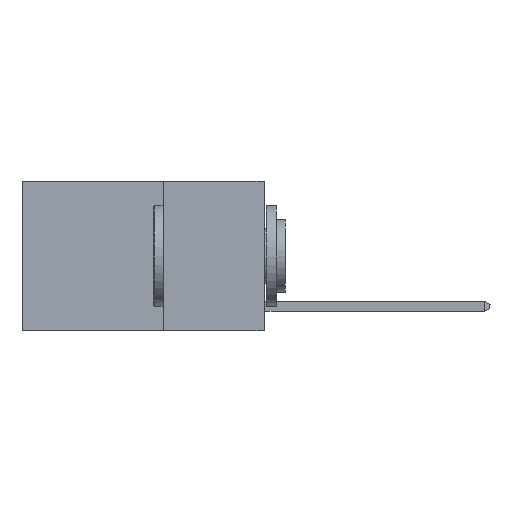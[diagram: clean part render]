
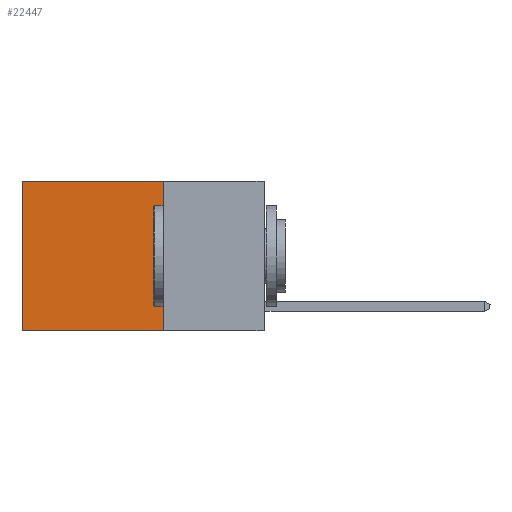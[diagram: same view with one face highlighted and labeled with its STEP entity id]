
A CAD part, left-side view. The second image highlights one B-rep face of the part: STEP entity #22447.
In plain terms, the highlighted planar face has unit normal (-1, 0, 0).
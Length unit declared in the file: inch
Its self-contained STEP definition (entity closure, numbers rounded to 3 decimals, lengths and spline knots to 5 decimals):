
#1353 = LINE ( 'NONE', #23215, #26452 ) ;
#2455 = DIRECTION ( 'NONE',  ( 0., 0., -1. ) ) ;
#3447 = VERTEX_POINT ( 'NONE', #26343 ) ;
#3857 = LINE ( 'NONE', #13785, #23564 ) ;
#3947 = DIRECTION ( 'NONE',  ( 0., 0., -1. ) ) ;
#5764 = VERTEX_POINT ( 'NONE', #14296 ) ;
#8653 = CARTESIAN_POINT ( 'NONE',  ( 0.2625, 0.25, 0. ) ) ;
#9069 = EDGE_CURVE ( 'NONE', #11595, #3447, #1353, .T. ) ;
#9349 = VECTOR ( 'NONE', #18840, 39.37008 ) ;
#10356 = VERTEX_POINT ( 'NONE', #8653 ) ;
#10792 = LINE ( 'NONE', #15302, #22115 ) ;
#11352 = FACE_OUTER_BOUND ( 'NONE', #25365, .T. ) ;
#11595 = VERTEX_POINT ( 'NONE', #27335 ) ;
#11889 = DIRECTION ( 'NONE',  ( 0., 0., -1. ) ) ;
#13785 = CARTESIAN_POINT ( 'NONE',  ( 0.2625, 0.25, 0. ) ) ;
#14296 = CARTESIAN_POINT ( 'NONE',  ( 0.2625, 0.6, 0. ) ) ;
#14953 = DIRECTION ( 'NONE',  ( 0., 1., 0. ) ) ;
#15302 = CARTESIAN_POINT ( 'NONE',  ( 0.2625, 0.6, 0. ) ) ;
#16429 = CARTESIAN_POINT ( 'NONE',  ( 0.2625, 0.25, 0. ) ) ;
#16587 = PLANE ( 'NONE',  #25099 ) ;
#16840 = ORIENTED_EDGE ( 'NONE', *, *, #21892, .T. ) ;
#18384 = LINE ( 'NONE', #16429, #9349 ) ;
#18714 = DIRECTION ( 'NONE',  ( 1., 0., 0. ) ) ;
#18840 = DIRECTION ( 'NONE',  ( 0., 1., 0. ) ) ;
#21737 = ORIENTED_EDGE ( 'NONE', *, *, #22923, .T. ) ;
#21892 = EDGE_CURVE ( 'NONE', #5764, #3447, #10792, .T. ) ;
#22115 = VECTOR ( 'NONE', #2455, 39.37008 ) ;
#22447 = ADVANCED_FACE ( 'NONE', ( #11352 ), #16587, .F. ) ;
#22923 = EDGE_CURVE ( 'NONE', #10356, #5764, #18384, .T. ) ;
#23084 = CARTESIAN_POINT ( 'NONE',  ( 0.2625, 0.25, 0. ) ) ;
#23215 = CARTESIAN_POINT ( 'NONE',  ( 0.2625, 0.25, -0.37 ) ) ;
#23564 = VECTOR ( 'NONE', #11889, 39.37008 ) ;
#25099 = AXIS2_PLACEMENT_3D ( 'NONE', #23084, #18714, #3947 ) ;
#25292 = EDGE_CURVE ( 'NONE', #10356, #11595, #3857, .T. ) ;
#25365 = EDGE_LOOP ( 'NONE', ( #16840, #26960, #27690, #21737 ) ) ;
#26343 = CARTESIAN_POINT ( 'NONE',  ( 0.2625, 0.6, -0.37 ) ) ;
#26452 = VECTOR ( 'NONE', #14953, 39.37008 ) ;
#26960 = ORIENTED_EDGE ( 'NONE', *, *, #9069, .F. ) ;
#27335 = CARTESIAN_POINT ( 'NONE',  ( 0.2625, 0.25, -0.37 ) ) ;
#27690 = ORIENTED_EDGE ( 'NONE', *, *, #25292, .F. ) ;
